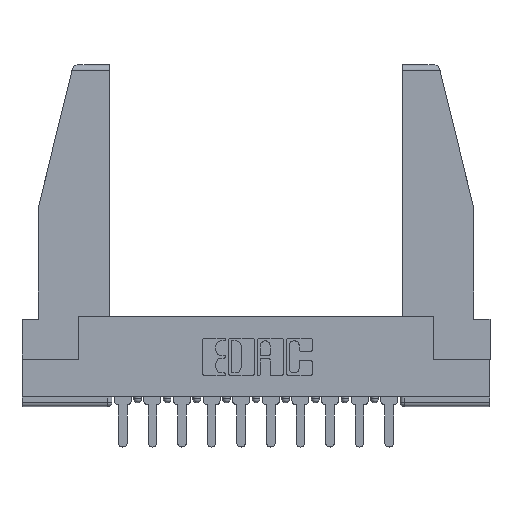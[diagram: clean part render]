
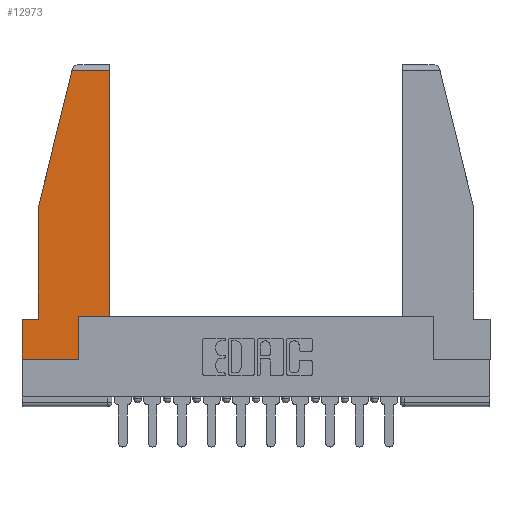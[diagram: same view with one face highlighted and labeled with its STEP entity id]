
A CAD part, top view. The second image highlights one B-rep face of the part: STEP entity #12973.
In plain terms, the highlighted planar face has unit normal (0, 0, 1).
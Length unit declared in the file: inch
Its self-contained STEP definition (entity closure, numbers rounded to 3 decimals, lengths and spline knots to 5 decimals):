
#64 = ORIENTED_EDGE ( 'NONE', *, *, #8236, .T. ) ;
#369 = ORIENTED_EDGE ( 'NONE', *, *, #1333, .T. ) ;
#456 = LINE ( 'NONE', #11978, #14724 ) ;
#586 = EDGE_CURVE ( 'NONE', #12816, #10543, #13505, .T. ) ;
#713 = CARTESIAN_POINT ( 'NONE',  ( 0., 1.52, 0. ) ) ;
#935 = ORIENTED_EDGE ( 'NONE', *, *, #3900, .T. ) ;
#1306 = DIRECTION ( 'NONE',  ( 0., -1., 0. ) ) ;
#1333 = EDGE_CURVE ( 'NONE', #4103, #12816, #11671, .T. ) ;
#1344 = VECTOR ( 'NONE', #8754, 39.37008 ) ;
#1392 = VECTOR ( 'NONE', #3582, 39.37008 ) ;
#2032 = VERTEX_POINT ( 'NONE', #12992 ) ;
#2075 = FACE_OUTER_BOUND ( 'NONE', #2720, .T. ) ;
#2714 = LINE ( 'NONE', #12446, #11590 ) ;
#2720 = EDGE_LOOP ( 'NONE', ( #9429, #4151, #369, #3239, #8376, #64, #8085, #935, #9559 ) ) ;
#2724 = PLANE ( 'NONE',  #14628 ) ;
#2778 = DIRECTION ( 'NONE',  ( 1., 0., 0. ) ) ;
#2890 = CARTESIAN_POINT ( 'NONE',  ( 0.086, 0.8, 0. ) ) ;
#2930 = DIRECTION ( 'NONE',  ( -1., 0., 0. ) ) ;
#3239 = ORIENTED_EDGE ( 'NONE', *, *, #586, .T. ) ;
#3287 = DIRECTION ( 'NONE',  ( 1., 0., 0. ) ) ;
#3370 = VERTEX_POINT ( 'NONE', #6682 ) ;
#3374 = CARTESIAN_POINT ( 'NONE',  ( 0.297, 0., 0. ) ) ;
#3582 = DIRECTION ( 'NONE',  ( 1., 0., 0. ) ) ;
#3900 = EDGE_CURVE ( 'NONE', #11237, #5025, #10875, .T. ) ;
#4103 = VERTEX_POINT ( 'NONE', #11849 ) ;
#4151 = ORIENTED_EDGE ( 'NONE', *, *, #8218, .T. ) ;
#4292 = CARTESIAN_POINT ( 'NONE',  ( 0., 0.21, 0. ) ) ;
#4428 = LINE ( 'NONE', #11061, #1344 ) ;
#4547 = EDGE_CURVE ( 'NONE', #3370, #11237, #8765, .T. ) ;
#4670 = LINE ( 'NONE', #4292, #10600 ) ;
#5025 = VERTEX_POINT ( 'NONE', #13894 ) ;
#5136 = DIRECTION ( 'NONE',  ( 0., 1., 0. ) ) ;
#5773 = CARTESIAN_POINT ( 'NONE',  ( 0., 0.21, 0. ) ) ;
#6682 = CARTESIAN_POINT ( 'NONE',  ( 0., 0., 0. ) ) ;
#6841 = VERTEX_POINT ( 'NONE', #5773 ) ;
#7033 = CARTESIAN_POINT ( 'NONE',  ( 0., 0., 0. ) ) ;
#7968 = CARTESIAN_POINT ( 'NONE',  ( 0.086, 0.21, 0. ) ) ;
#8085 = ORIENTED_EDGE ( 'NONE', *, *, #4547, .T. ) ;
#8218 = EDGE_CURVE ( 'NONE', #14853, #4103, #13632, .T. ) ;
#8236 = EDGE_CURVE ( 'NONE', #6841, #3370, #4428, .T. ) ;
#8376 = ORIENTED_EDGE ( 'NONE', *, *, #11924, .T. ) ;
#8551 = VECTOR ( 'NONE', #10406, 39.37008 ) ;
#8604 = DIRECTION ( 'NONE',  ( 0., 0., 1. ) ) ;
#8754 = DIRECTION ( 'NONE',  ( 0., -1., 0. ) ) ;
#8765 = LINE ( 'NONE', #7033, #1392 ) ;
#9429 = ORIENTED_EDGE ( 'NONE', *, *, #12986, .T. ) ;
#9524 = CARTESIAN_POINT ( 'NONE',  ( 0.086, 0.8, 0. ) ) ;
#9559 = ORIENTED_EDGE ( 'NONE', *, *, #10629, .T. ) ;
#10406 = DIRECTION ( 'NONE',  ( -0.239, -0.971, 0. ) ) ;
#10543 = VERTEX_POINT ( 'NONE', #7968 ) ;
#10600 = VECTOR ( 'NONE', #14784, 39.37008 ) ;
#10629 = EDGE_CURVE ( 'NONE', #5025, #2032, #2714, .T. ) ;
#10776 = VECTOR ( 'NONE', #1306, 39.37008 ) ;
#10815 = CARTESIAN_POINT ( 'NONE',  ( 0., 0., 0. ) ) ;
#10875 = LINE ( 'NONE', #3374, #12153 ) ;
#11061 = CARTESIAN_POINT ( 'NONE',  ( 0., 0.21, 0. ) ) ;
#11105 = VECTOR ( 'NONE', #2930, 39.37008 ) ;
#11237 = VERTEX_POINT ( 'NONE', #13424 ) ;
#11590 = VECTOR ( 'NONE', #3287, 39.37008 ) ;
#11671 = LINE ( 'NONE', #14285, #8551 ) ;
#11849 = CARTESIAN_POINT ( 'NONE',  ( 0.2636, 1.52, 0. ) ) ;
#11924 = EDGE_CURVE ( 'NONE', #10543, #6841, #4670, .T. ) ;
#11978 = CARTESIAN_POINT ( 'NONE',  ( 0.461, 0.223, 0. ) ) ;
#12153 = VECTOR ( 'NONE', #13788, 39.37008 ) ;
#12446 = CARTESIAN_POINT ( 'NONE',  ( 0.297, 0.223, 0. ) ) ;
#12816 = VERTEX_POINT ( 'NONE', #9524 ) ;
#12973 = ADVANCED_FACE ( 'NONE', ( #2075 ), #2724, .T. ) ;
#12986 = EDGE_CURVE ( 'NONE', #2032, #14853, #456, .T. ) ;
#12992 = CARTESIAN_POINT ( 'NONE',  ( 0.461, 0.223, 0. ) ) ;
#13424 = CARTESIAN_POINT ( 'NONE',  ( 0.297, 0., 0. ) ) ;
#13505 = LINE ( 'NONE', #2890, #10776 ) ;
#13632 = LINE ( 'NONE', #713, #11105 ) ;
#13788 = DIRECTION ( 'NONE',  ( 0., 1., 0. ) ) ;
#13894 = CARTESIAN_POINT ( 'NONE',  ( 0.297, 0.223, 0. ) ) ;
#14285 = CARTESIAN_POINT ( 'NONE',  ( 0.271, 1.55, 0. ) ) ;
#14526 = CARTESIAN_POINT ( 'NONE',  ( 0.461, 1.52, 0. ) ) ;
#14628 = AXIS2_PLACEMENT_3D ( 'NONE', #10815, #8604, #2778 ) ;
#14724 = VECTOR ( 'NONE', #5136, 39.37008 ) ;
#14784 = DIRECTION ( 'NONE',  ( -1., 0., 0. ) ) ;
#14853 = VERTEX_POINT ( 'NONE', #14526 ) ;
